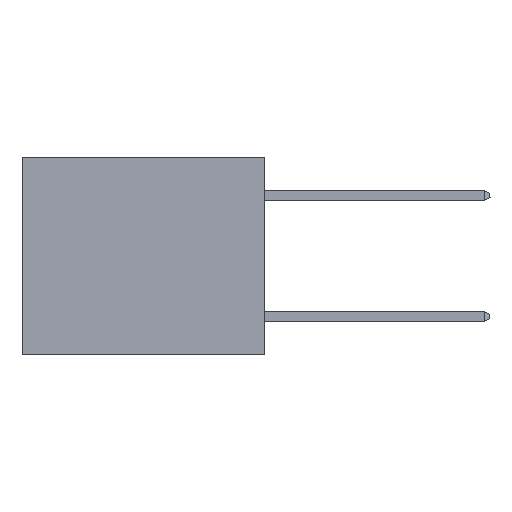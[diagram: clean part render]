
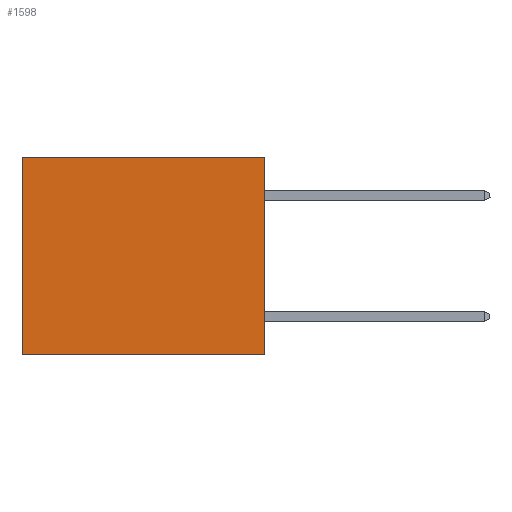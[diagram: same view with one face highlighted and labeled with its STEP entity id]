
A CAD part, left-side view. The second image highlights one B-rep face of the part: STEP entity #1598.
In plain terms, the highlighted planar face has unit normal (-1, 0, 0).
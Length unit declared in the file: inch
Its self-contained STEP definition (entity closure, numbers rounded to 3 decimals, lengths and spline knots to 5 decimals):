
#1196 = DIRECTION ( 'NONE',  ( 0., 0., -1. ) ) ;
#1375 = VECTOR ( 'NONE', #22817, 39.37008 ) ;
#1598 = ADVANCED_FACE ( 'NONE', ( #25613 ), #3310, .F. ) ;
#1881 = VECTOR ( 'NONE', #1196, 39.37008 ) ;
#2827 = CARTESIAN_POINT ( 'NONE',  ( 0.3165, 0., -0.49 ) ) ;
#3310 = PLANE ( 'NONE',  #10251 ) ;
#4572 = CARTESIAN_POINT ( 'NONE',  ( 0.3165, 0.6, 0. ) ) ;
#5337 = CARTESIAN_POINT ( 'NONE',  ( 0.3165, 0., -0.49 ) ) ;
#5562 = ORIENTED_EDGE ( 'NONE', *, *, #8008, .T. ) ;
#5665 = ORIENTED_EDGE ( 'NONE', *, *, #11957, .F. ) ;
#5847 = DIRECTION ( 'NONE',  ( 1., 0., 0. ) ) ;
#5852 = LINE ( 'NONE', #2827, #15158 ) ;
#6719 = DIRECTION ( 'NONE',  ( 0., 0., -1. ) ) ;
#8008 = EDGE_CURVE ( 'NONE', #14108, #12543, #22455, .T. ) ;
#8958 = VERTEX_POINT ( 'NONE', #14904 ) ;
#9000 = LINE ( 'NONE', #13094, #1881 ) ;
#10171 = CARTESIAN_POINT ( 'NONE',  ( 0.3165, 0., -0.49 ) ) ;
#10251 = AXIS2_PLACEMENT_3D ( 'NONE', #5337, #5847, #17981 ) ;
#11182 = ORIENTED_EDGE ( 'NONE', *, *, #21997, .T. ) ;
#11957 = EDGE_CURVE ( 'NONE', #19709, #12543, #5852, .T. ) ;
#12543 = VERTEX_POINT ( 'NONE', #24400 ) ;
#13094 = CARTESIAN_POINT ( 'NONE',  ( 0.3165, 0., -0.49 ) ) ;
#14108 = VERTEX_POINT ( 'NONE', #4572 ) ;
#14553 = DIRECTION ( 'NONE',  ( 0., 1., 0. ) ) ;
#14904 = CARTESIAN_POINT ( 'NONE',  ( 0.3165, 0., 0. ) ) ;
#15158 = VECTOR ( 'NONE', #14553, 39.37008 ) ;
#15679 = LINE ( 'NONE', #17010, #1375 ) ;
#17010 = CARTESIAN_POINT ( 'NONE',  ( 0.3165, 0., 0. ) ) ;
#17981 = DIRECTION ( 'NONE',  ( 0., 0., -1. ) ) ;
#18268 = EDGE_CURVE ( 'NONE', #8958, #19709, #9000, .T. ) ;
#19709 = VERTEX_POINT ( 'NONE', #10171 ) ;
#21895 = EDGE_LOOP ( 'NONE', ( #5562, #5665, #23842, #11182 ) ) ;
#21997 = EDGE_CURVE ( 'NONE', #8958, #14108, #15679, .T. ) ;
#22455 = LINE ( 'NONE', #24611, #25606 ) ;
#22817 = DIRECTION ( 'NONE',  ( 0., 1., 0. ) ) ;
#23842 = ORIENTED_EDGE ( 'NONE', *, *, #18268, .F. ) ;
#24400 = CARTESIAN_POINT ( 'NONE',  ( 0.3165, 0.6, -0.49 ) ) ;
#24611 = CARTESIAN_POINT ( 'NONE',  ( 0.3165, 0.6, -0.49 ) ) ;
#25606 = VECTOR ( 'NONE', #6719, 39.37008 ) ;
#25613 = FACE_OUTER_BOUND ( 'NONE', #21895, .T. ) ;
